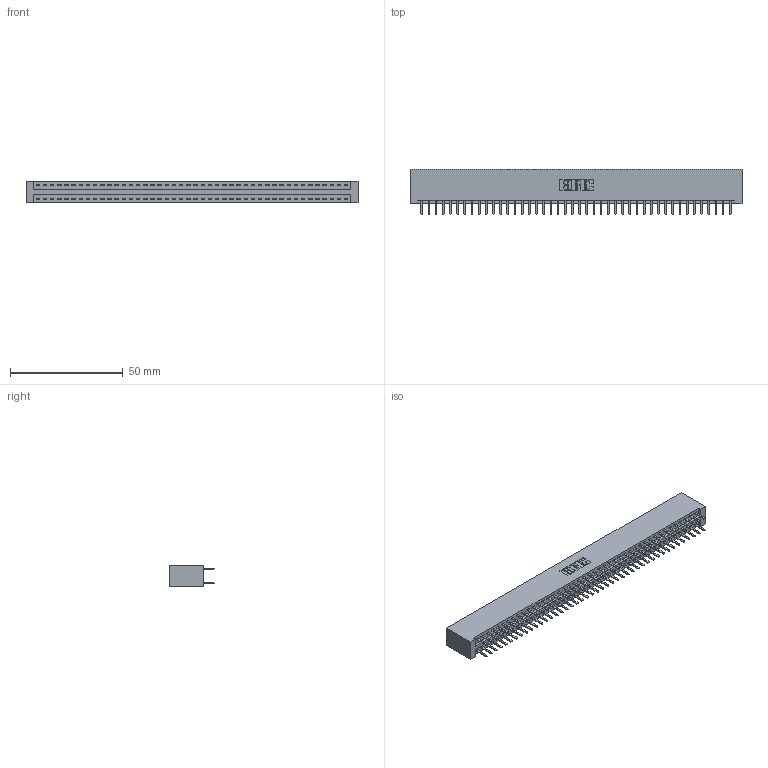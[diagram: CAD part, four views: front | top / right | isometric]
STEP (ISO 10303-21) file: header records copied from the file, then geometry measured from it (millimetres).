
FILE_DESCRIPTION (( 'STEP AP203' ), '1' );
FILE_NAME ('396-088-520-201.STEP', '2019-10-31T01:00:19', ( '' ), ( '' ), 'SwSTEP 2.0', 'SolidWorks 2016', '' );
FILE_SCHEMA (( 'CONFIG_CONTROL_DESIGN' ));
Length unit declared in the file: inch
Products named in the file (3): 345-292-001_345-293-120; 396-088-520-201; 346 Part_No Mounting Lugs
Assembly tree (89 placements, depth 2):
  396-088-520-201
    346 Part_No Mounting Lugs
    345-292-001_345-293-120  x88
Bounding box: 146.94 x 20.02 x 9.4 mm (x, y, z)
Volume: 14878.5 mm3; surface area: 20555.5 mm2
Topology: 89 solids, 89 shells, 5042 faces, 14649 edges, 9530 vertices
Faces by surface type: plane 3328, cylinder 1714
Entity records: 28283 total; most frequent: CARTESIAN_POINT 4668, ORIENTED_EDGE 4590, DIRECTION 4147, EDGE_CURVE 2295, VECTOR 1991, LINE 1991, VERTEX_POINT 1526, AXIS2_PLACEMENT_3D 1078
